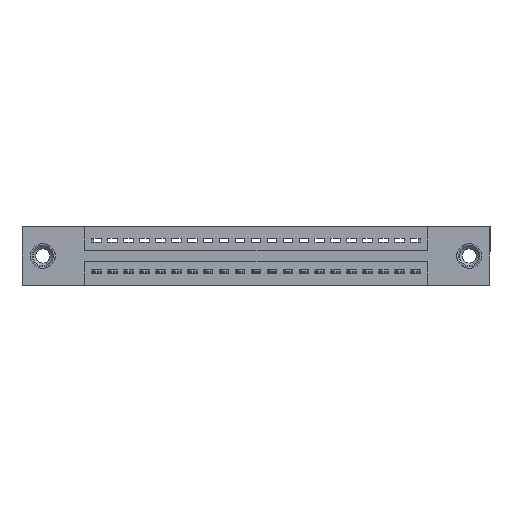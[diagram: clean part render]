
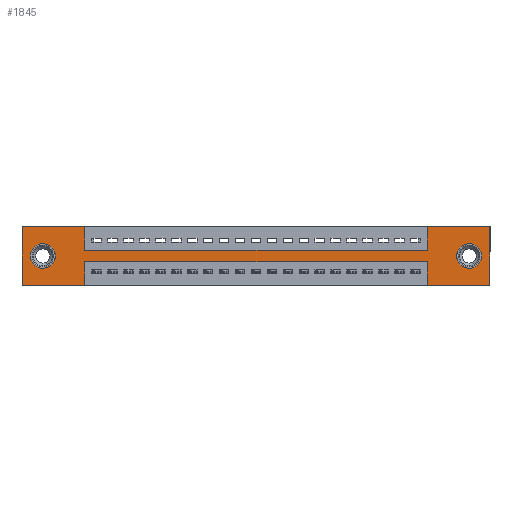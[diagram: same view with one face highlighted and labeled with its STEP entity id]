
A CAD part, front view. The second image highlights one B-rep face of the part: STEP entity #1845.
In plain terms, the highlighted planar face has unit normal (0, -1, 0).
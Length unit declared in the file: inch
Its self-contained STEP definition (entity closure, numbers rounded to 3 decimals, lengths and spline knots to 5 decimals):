
#352 = VECTOR ( 'NONE', #959, 39.37008 ) ;
#371 = CIRCLE ( 'NONE', #6656, 0.078 ) ;
#959 = DIRECTION ( 'NONE',  ( 0., 0., -1. ) ) ;
#1090 = FACE_OUTER_BOUND ( 'NONE', #17199, .T. ) ;
#1223 = DIRECTION ( 'NONE',  ( 0., 0., -1. ) ) ;
#1300 = VECTOR ( 'NONE', #1803, 39.37008 ) ;
#1353 = DIRECTION ( 'NONE',  ( 0., 1., 0. ) ) ;
#1401 = VECTOR ( 'NONE', #18736, 39.37008 ) ;
#1651 = CARTESIAN_POINT ( 'NONE',  ( 0., 0., -0.37 ) ) ;
#1684 = VECTOR ( 'NONE', #13964, 39.37008 ) ;
#1803 = DIRECTION ( 'NONE',  ( 1., 0., 0. ) ) ;
#1845 = ADVANCED_FACE ( 'NONE', ( #16877, #12593, #1090 ), #16973, .T. ) ;
#1996 = VERTEX_POINT ( 'NONE', #11144 ) ;
#2011 = CARTESIAN_POINT ( 'NONE',  ( 0.3925, 0., 0. ) ) ;
#2169 = VERTEX_POINT ( 'NONE', #2011 ) ;
#2366 = AXIS2_PLACEMENT_3D ( 'NONE', #14167, #1353, #11030 ) ;
#2616 = VERTEX_POINT ( 'NONE', #12755 ) ;
#3119 = EDGE_LOOP ( 'NONE', ( #4627, #13562 ) ) ;
#3442 = VERTEX_POINT ( 'NONE', #7589 ) ;
#3490 = DIRECTION ( 'NONE',  ( 0., 0., 1. ) ) ;
#3658 = VERTEX_POINT ( 'NONE', #4580 ) ;
#3759 = CARTESIAN_POINT ( 'NONE',  ( 0.3925, 0., -0.15 ) ) ;
#3950 = ORIENTED_EDGE ( 'NONE', *, *, #9979, .F. ) ;
#3971 = AXIS2_PLACEMENT_3D ( 'NONE', #20146, #15331, #13800 ) ;
#4019 = DIRECTION ( 'NONE',  ( 0., -1., 0. ) ) ;
#4087 = CIRCLE ( 'NONE', #12993, 0.078 ) ;
#4141 = CARTESIAN_POINT ( 'NONE',  ( 0., 0., 0. ) ) ;
#4281 = ORIENTED_EDGE ( 'NONE', *, *, #15914, .F. ) ;
#4320 = CARTESIAN_POINT ( 'NONE',  ( 0.3925, 0., 0. ) ) ;
#4580 = CARTESIAN_POINT ( 'NONE',  ( 2.935, 0., 0. ) ) ;
#4627 = ORIENTED_EDGE ( 'NONE', *, *, #17127, .T. ) ;
#4712 = ORIENTED_EDGE ( 'NONE', *, *, #15748, .F. ) ;
#5099 = CARTESIAN_POINT ( 'NONE',  ( 2.5425, 0., -0.37 ) ) ;
#5233 = CARTESIAN_POINT ( 'NONE',  ( 2.5425, 0., 0. ) ) ;
#5235 = ORIENTED_EDGE ( 'NONE', *, *, #16579, .F. ) ;
#5357 = ORIENTED_EDGE ( 'NONE', *, *, #5466, .F. ) ;
#5466 = EDGE_CURVE ( 'NONE', #18187, #17329, #18663, .T. ) ;
#5775 = VERTEX_POINT ( 'NONE', #19035 ) ;
#5862 = EDGE_CURVE ( 'NONE', #19631, #2169, #12575, .T. ) ;
#5975 = CARTESIAN_POINT ( 'NONE',  ( 0., 0., -0.37 ) ) ;
#6505 = CARTESIAN_POINT ( 'NONE',  ( 0.3925, 0., -0.15 ) ) ;
#6510 = CARTESIAN_POINT ( 'NONE',  ( 2.935, 0., 0. ) ) ;
#6555 = ORIENTED_EDGE ( 'NONE', *, *, #18507, .F. ) ;
#6591 = DIRECTION ( 'NONE',  ( 0., 0., -1. ) ) ;
#6656 = AXIS2_PLACEMENT_3D ( 'NONE', #16703, #18336, #13602 ) ;
#6901 = ORIENTED_EDGE ( 'NONE', *, *, #7178, .T. ) ;
#6987 = VECTOR ( 'NONE', #16020, 39.37008 ) ;
#7014 = VECTOR ( 'NONE', #15516, 39.37008 ) ;
#7172 = ORIENTED_EDGE ( 'NONE', *, *, #17264, .T. ) ;
#7178 = EDGE_CURVE ( 'NONE', #5775, #7819, #20580, .T. ) ;
#7533 = VERTEX_POINT ( 'NONE', #19161 ) ;
#7583 = DIRECTION ( 'NONE',  ( -1., 0., 0. ) ) ;
#7589 = CARTESIAN_POINT ( 'NONE',  ( 0.13, 0., -0.263 ) ) ;
#7819 = VERTEX_POINT ( 'NONE', #12641 ) ;
#8300 = DIRECTION ( 'NONE',  ( 0., 0., 1. ) ) ;
#8391 = EDGE_CURVE ( 'NONE', #16716, #3658, #14440, .T. ) ;
#8517 = CARTESIAN_POINT ( 'NONE',  ( 2.5425, 0., -0.15 ) ) ;
#8724 = VECTOR ( 'NONE', #1223, 39.37008 ) ;
#8912 = CARTESIAN_POINT ( 'NONE',  ( 0., 0., 0. ) ) ;
#8937 = CARTESIAN_POINT ( 'NONE',  ( 0., 0., -0.37 ) ) ;
#9476 = ORIENTED_EDGE ( 'NONE', *, *, #12153, .F. ) ;
#9604 = DIRECTION ( 'NONE',  ( 0., 1., 0. ) ) ;
#9979 = EDGE_CURVE ( 'NONE', #3658, #7533, #19917, .T. ) ;
#10077 = ORIENTED_EDGE ( 'NONE', *, *, #8391, .F. ) ;
#10529 = EDGE_CURVE ( 'NONE', #3442, #1996, #4087, .T. ) ;
#10573 = CARTESIAN_POINT ( 'NONE',  ( 0.3925, 0., -0.22 ) ) ;
#10903 = CARTESIAN_POINT ( 'NONE',  ( 0.3925, 0., -0.37 ) ) ;
#11030 = DIRECTION ( 'NONE',  ( 0., 0., -1. ) ) ;
#11038 = CARTESIAN_POINT ( 'NONE',  ( 0.3925, 0., -0.22 ) ) ;
#11144 = CARTESIAN_POINT ( 'NONE',  ( 0.13, 0., -0.107 ) ) ;
#11479 = EDGE_CURVE ( 'NONE', #17329, #16716, #17082, .T. ) ;
#11496 = LINE ( 'NONE', #1651, #6987 ) ;
#11829 = DIRECTION ( 'NONE',  ( 0., 0., 1. ) ) ;
#11919 = CARTESIAN_POINT ( 'NONE',  ( 0., 0., 0. ) ) ;
#12033 = LINE ( 'NONE', #10573, #7014 ) ;
#12074 = DIRECTION ( 'NONE',  ( 0., 0., -1. ) ) ;
#12153 = EDGE_CURVE ( 'NONE', #16696, #13518, #12033, .T. ) ;
#12559 = ORIENTED_EDGE ( 'NONE', *, *, #13185, .F. ) ;
#12575 = LINE ( 'NONE', #14417, #1300 ) ;
#12593 = FACE_BOUND ( 'NONE', #3119, .T. ) ;
#12641 = CARTESIAN_POINT ( 'NONE',  ( 2.805, 0., -0.107 ) ) ;
#12755 = CARTESIAN_POINT ( 'NONE',  ( 2.5425, 0., -0.37 ) ) ;
#12993 = AXIS2_PLACEMENT_3D ( 'NONE', #19248, #9604, #11829 ) ;
#13185 = EDGE_CURVE ( 'NONE', #13518, #18003, #20787, .T. ) ;
#13518 = VERTEX_POINT ( 'NONE', #11038 ) ;
#13562 = ORIENTED_EDGE ( 'NONE', *, *, #10529, .T. ) ;
#13602 = DIRECTION ( 'NONE',  ( 0., 0., 1. ) ) ;
#13800 = DIRECTION ( 'NONE',  ( 0., 0., -1. ) ) ;
#13873 = VECTOR ( 'NONE', #6591, 39.37008 ) ;
#13964 = DIRECTION ( 'NONE',  ( 0., 0., 1. ) ) ;
#14040 = LINE ( 'NONE', #5975, #14789 ) ;
#14167 = CARTESIAN_POINT ( 'NONE',  ( 2.805, 0., -0.185 ) ) ;
#14353 = VECTOR ( 'NONE', #16512, 39.37008 ) ;
#14417 = CARTESIAN_POINT ( 'NONE',  ( 0., 0., 0. ) ) ;
#14440 = LINE ( 'NONE', #4141, #1401 ) ;
#14671 = EDGE_CURVE ( 'NONE', #7533, #2616, #14040, .T. ) ;
#14789 = VECTOR ( 'NONE', #7583, 39.37008 ) ;
#15054 = EDGE_LOOP ( 'NONE', ( #7172, #6901 ) ) ;
#15331 = DIRECTION ( 'NONE',  ( 0., 1., 0. ) ) ;
#15516 = DIRECTION ( 'NONE',  ( -1., 0., 0. ) ) ;
#15748 = EDGE_CURVE ( 'NONE', #18003, #18531, #11496, .T. ) ;
#15914 = EDGE_CURVE ( 'NONE', #18531, #19631, #18789, .T. ) ;
#16020 = DIRECTION ( 'NONE',  ( -1., 0., 0. ) ) ;
#16047 = CARTESIAN_POINT ( 'NONE',  ( 0.3925, 0., -0.37 ) ) ;
#16255 = ORIENTED_EDGE ( 'NONE', *, *, #5862, .F. ) ;
#16512 = DIRECTION ( 'NONE',  ( 1., 0., 0. ) ) ;
#16579 = EDGE_CURVE ( 'NONE', #2616, #16696, #19272, .T. ) ;
#16696 = VERTEX_POINT ( 'NONE', #20267 ) ;
#16703 = CARTESIAN_POINT ( 'NONE',  ( 0.13, 0., -0.185 ) ) ;
#16716 = VERTEX_POINT ( 'NONE', #17078 ) ;
#16877 = FACE_BOUND ( 'NONE', #15054, .T. ) ;
#16973 = PLANE ( 'NONE',  #20166 ) ;
#17078 = CARTESIAN_POINT ( 'NONE',  ( 2.5425, 0., 0. ) ) ;
#17082 = LINE ( 'NONE', #5233, #19621 ) ;
#17127 = EDGE_CURVE ( 'NONE', #1996, #3442, #371, .T. ) ;
#17199 = EDGE_LOOP ( 'NONE', ( #12559, #9476, #5235, #19167, #3950, #10077, #20749, #5357, #6555, #16255, #4281, #4712 ) ) ;
#17264 = EDGE_CURVE ( 'NONE', #7819, #5775, #20728, .T. ) ;
#17329 = VERTEX_POINT ( 'NONE', #8517 ) ;
#18003 = VERTEX_POINT ( 'NONE', #16047 ) ;
#18187 = VERTEX_POINT ( 'NONE', #6505 ) ;
#18336 = DIRECTION ( 'NONE',  ( 0., 1., 0. ) ) ;
#18507 = EDGE_CURVE ( 'NONE', #2169, #18187, #19702, .T. ) ;
#18531 = VERTEX_POINT ( 'NONE', #8937 ) ;
#18663 = LINE ( 'NONE', #3759, #14353 ) ;
#18736 = DIRECTION ( 'NONE',  ( 1., 0., 0. ) ) ;
#18789 = LINE ( 'NONE', #8912, #1684 ) ;
#19020 = VECTOR ( 'NONE', #3490, 39.37008 ) ;
#19035 = CARTESIAN_POINT ( 'NONE',  ( 2.805, 0., -0.263 ) ) ;
#19161 = CARTESIAN_POINT ( 'NONE',  ( 2.935, 0., -0.37 ) ) ;
#19167 = ORIENTED_EDGE ( 'NONE', *, *, #14671, .F. ) ;
#19248 = CARTESIAN_POINT ( 'NONE',  ( 0.13, 0., -0.185 ) ) ;
#19272 = LINE ( 'NONE', #5099, #19020 ) ;
#19621 = VECTOR ( 'NONE', #8300, 39.37008 ) ;
#19631 = VERTEX_POINT ( 'NONE', #11919 ) ;
#19702 = LINE ( 'NONE', #4320, #352 ) ;
#19917 = LINE ( 'NONE', #6510, #13873 ) ;
#20146 = CARTESIAN_POINT ( 'NONE',  ( 2.805, 0., -0.185 ) ) ;
#20166 = AXIS2_PLACEMENT_3D ( 'NONE', #20230, #4019, #12074 ) ;
#20230 = CARTESIAN_POINT ( 'NONE',  ( 0., 0., -0.37 ) ) ;
#20267 = CARTESIAN_POINT ( 'NONE',  ( 2.5425, 0., -0.22 ) ) ;
#20580 = CIRCLE ( 'NONE', #2366, 0.078 ) ;
#20728 = CIRCLE ( 'NONE', #3971, 0.078 ) ;
#20749 = ORIENTED_EDGE ( 'NONE', *, *, #11479, .F. ) ;
#20787 = LINE ( 'NONE', #10903, #8724 ) ;
